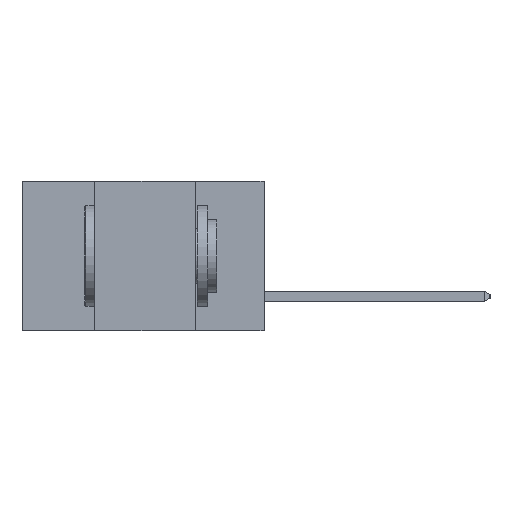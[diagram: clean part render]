
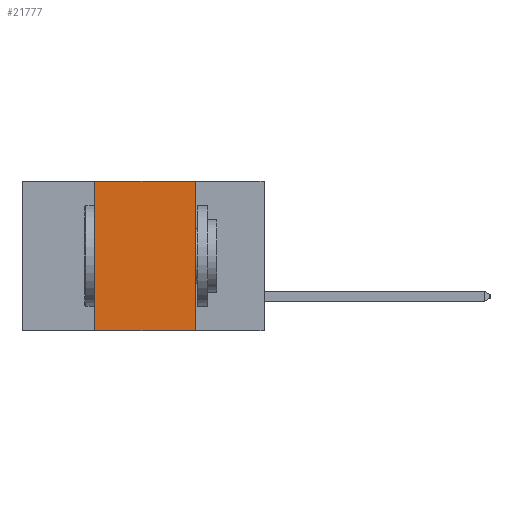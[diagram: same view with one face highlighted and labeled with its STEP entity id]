
A CAD part, left-side view. The second image highlights one B-rep face of the part: STEP entity #21777.
In plain terms, the highlighted planar face has unit normal (-1, 0, 0).
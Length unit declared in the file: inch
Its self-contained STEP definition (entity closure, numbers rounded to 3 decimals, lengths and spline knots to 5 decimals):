
#1631 = VERTEX_POINT ( 'NONE', #9658 ) ;
#2139 = LINE ( 'NONE', #6599, #11063 ) ;
#2269 = CARTESIAN_POINT ( 'NONE',  ( 0., 0.17, 0. ) ) ;
#2462 = VERTEX_POINT ( 'NONE', #19311 ) ;
#3200 = ORIENTED_EDGE ( 'NONE', *, *, #19283, .F. ) ;
#4164 = LINE ( 'NONE', #18347, #4728 ) ;
#4728 = VECTOR ( 'NONE', #18556, 39.37008 ) ;
#5733 = CARTESIAN_POINT ( 'NONE',  ( 0., 0.17, -0.37 ) ) ;
#6506 = VERTEX_POINT ( 'NONE', #2269 ) ;
#6599 = CARTESIAN_POINT ( 'NONE',  ( 0., 0.42, -0.37 ) ) ;
#6888 = ORIENTED_EDGE ( 'NONE', *, *, #21530, .T. ) ;
#7606 = CARTESIAN_POINT ( 'NONE',  ( 0., 0.6, -0.37 ) ) ;
#7697 = LINE ( 'NONE', #7606, #16425 ) ;
#8368 = PLANE ( 'NONE',  #13244 ) ;
#9350 = DIRECTION ( 'NONE',  ( 0., -1., 0. ) ) ;
#9658 = CARTESIAN_POINT ( 'NONE',  ( 0., 0.42, 0. ) ) ;
#9795 = DIRECTION ( 'NONE',  ( 0., 0., -1. ) ) ;
#9977 = EDGE_LOOP ( 'NONE', ( #19980, #10184, #3200, #6888 ) ) ;
#10099 = DIRECTION ( 'NONE',  ( 0., 0., -1. ) ) ;
#10184 = ORIENTED_EDGE ( 'NONE', *, *, #18114, .F. ) ;
#10890 = CARTESIAN_POINT ( 'NONE',  ( 0., 0.17, -0.37 ) ) ;
#11063 = VECTOR ( 'NONE', #11889, 39.37008 ) ;
#11889 = DIRECTION ( 'NONE',  ( 0., 0., 1. ) ) ;
#13244 = AXIS2_PLACEMENT_3D ( 'NONE', #13552, #20483, #10099 ) ;
#13552 = CARTESIAN_POINT ( 'NONE',  ( 0., 0.6, 0. ) ) ;
#14285 = VERTEX_POINT ( 'NONE', #5733 ) ;
#14656 = EDGE_CURVE ( 'NONE', #6506, #14285, #14733, .T. ) ;
#14733 = LINE ( 'NONE', #10890, #18769 ) ;
#16425 = VECTOR ( 'NONE', #9350, 39.37008 ) ;
#18018 = FACE_OUTER_BOUND ( 'NONE', #9977, .T. ) ;
#18114 = EDGE_CURVE ( 'NONE', #1631, #6506, #4164, .T. ) ;
#18347 = CARTESIAN_POINT ( 'NONE',  ( 0., 0.6, 0. ) ) ;
#18556 = DIRECTION ( 'NONE',  ( 0., -1., 0. ) ) ;
#18769 = VECTOR ( 'NONE', #9795, 39.37008 ) ;
#19283 = EDGE_CURVE ( 'NONE', #2462, #1631, #2139, .T. ) ;
#19311 = CARTESIAN_POINT ( 'NONE',  ( 0., 0.42, -0.37 ) ) ;
#19980 = ORIENTED_EDGE ( 'NONE', *, *, #14656, .F. ) ;
#20483 = DIRECTION ( 'NONE',  ( 1., 0., 0. ) ) ;
#21530 = EDGE_CURVE ( 'NONE', #2462, #14285, #7697, .T. ) ;
#21777 = ADVANCED_FACE ( 'NONE', ( #18018 ), #8368, .F. ) ;
